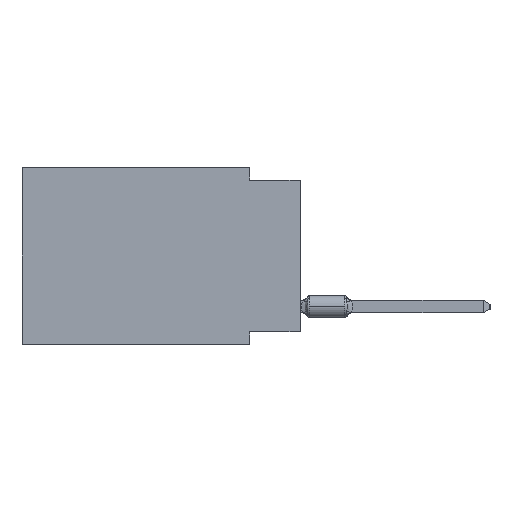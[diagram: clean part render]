
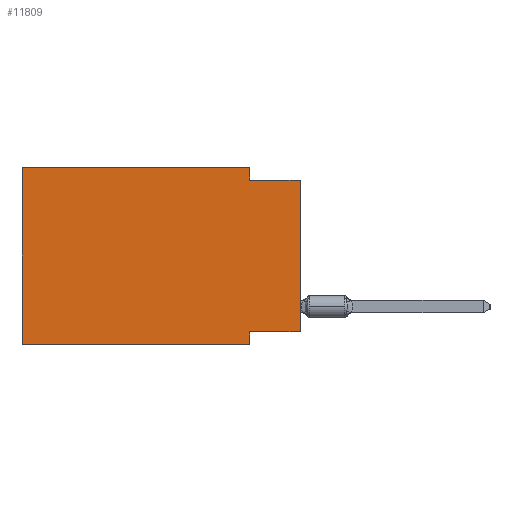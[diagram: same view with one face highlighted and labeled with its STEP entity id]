
A CAD part, left-side view. The second image highlights one B-rep face of the part: STEP entity #11809.
In plain terms, the highlighted planar face has unit normal (-1, 0, 0).
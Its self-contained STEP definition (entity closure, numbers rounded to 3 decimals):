
#423 = VECTOR ( 'NONE', #34263, 1000. ) ;
#4554 = CARTESIAN_POINT ( 'NONE',  ( 0., 2.54, -0.635 ) ) ;
#5944 = CARTESIAN_POINT ( 'NONE',  ( 0., 0., -8.255 ) ) ;
#6175 = VERTEX_POINT ( 'NONE', #35856 ) ;
#7278 = DIRECTION ( 'NONE',  ( 1., 0., 0. ) ) ;
#7930 = CARTESIAN_POINT ( 'NONE',  ( 0., 0., 0. ) ) ;
#10814 = CARTESIAN_POINT ( 'NONE',  ( 0., 13.97, 0. ) ) ;
#11542 = PLANE ( 'NONE',  #63949 ) ;
#11809 = ADVANCED_FACE ( 'NONE', ( #55339 ), #11542, .F. ) ;
#11859 = ORIENTED_EDGE ( 'NONE', *, *, #68750, .T. ) ;
#13327 = DIRECTION ( 'NONE',  ( 0., -1., 0. ) ) ;
#14011 = CARTESIAN_POINT ( 'NONE',  ( 0., 2.54, -8.89 ) ) ;
#14726 = VERTEX_POINT ( 'NONE', #75364 ) ;
#15876 = VECTOR ( 'NONE', #23024, 1000. ) ;
#18136 = VERTEX_POINT ( 'NONE', #66892 ) ;
#18162 = EDGE_CURVE ( 'NONE', #73712, #54810, #82327, .T. ) ;
#18544 = EDGE_CURVE ( 'NONE', #6175, #18136, #63864, .T. ) ;
#19356 = ORIENTED_EDGE ( 'NONE', *, *, #59135, .F. ) ;
#19653 = CARTESIAN_POINT ( 'NONE',  ( 0., 2.54, 0. ) ) ;
#20733 = VECTOR ( 'NONE', #71920, 1000. ) ;
#21104 = CARTESIAN_POINT ( 'NONE',  ( 0., 13.97, 0. ) ) ;
#21625 = VERTEX_POINT ( 'NONE', #33904 ) ;
#22103 = LINE ( 'NONE', #7930, #15876 ) ;
#22720 = CARTESIAN_POINT ( 'NONE',  ( 0., 2.54, 0. ) ) ;
#23024 = DIRECTION ( 'NONE',  ( 0., 0., 1. ) ) ;
#26619 = EDGE_CURVE ( 'NONE', #26950, #73712, #61394, .T. ) ;
#26950 = VERTEX_POINT ( 'NONE', #10814 ) ;
#27427 = CARTESIAN_POINT ( 'NONE',  ( 0., 13.97, 0. ) ) ;
#28576 = VECTOR ( 'NONE', #75507, 1000. ) ;
#33072 = VECTOR ( 'NONE', #49241, 1000. ) ;
#33843 = LINE ( 'NONE', #5944, #68025 ) ;
#33904 = CARTESIAN_POINT ( 'NONE',  ( 0., 13.97, -8.89 ) ) ;
#34263 = DIRECTION ( 'NONE',  ( 0., 0., -1. ) ) ;
#35721 = ORIENTED_EDGE ( 'NONE', *, *, #18162, .F. ) ;
#35856 = CARTESIAN_POINT ( 'NONE',  ( 0., 2.54, -8.255 ) ) ;
#38516 = VECTOR ( 'NONE', #90359, 1000. ) ;
#39804 = CARTESIAN_POINT ( 'NONE',  ( 0., 13.97, 0. ) ) ;
#40268 = LINE ( 'NONE', #39804, #28576 ) ;
#48632 = ORIENTED_EDGE ( 'NONE', *, *, #78523, .F. ) ;
#49241 = DIRECTION ( 'NONE',  ( 0., 0., -1. ) ) ;
#52419 = EDGE_CURVE ( 'NONE', #14726, #77624, #22103, .T. ) ;
#54810 = VERTEX_POINT ( 'NONE', #4554 ) ;
#55339 = FACE_OUTER_BOUND ( 'NONE', #86057, .T. ) ;
#57518 = VECTOR ( 'NONE', #13327, 1000. ) ;
#59098 = EDGE_CURVE ( 'NONE', #14726, #6175, #33843, .T. ) ;
#59135 = EDGE_CURVE ( 'NONE', #21625, #26950, #40268, .T. ) ;
#59907 = CARTESIAN_POINT ( 'NONE',  ( 0., 0., -0.635 ) ) ;
#60044 = DIRECTION ( 'NONE',  ( 0., 0., -1. ) ) ;
#61062 = CARTESIAN_POINT ( 'NONE',  ( 0., 13.97, -8.89 ) ) ;
#61394 = LINE ( 'NONE', #21104, #57518 ) ;
#63864 = LINE ( 'NONE', #14011, #33072 ) ;
#63949 = AXIS2_PLACEMENT_3D ( 'NONE', #27427, #7278, #60044 ) ;
#66892 = CARTESIAN_POINT ( 'NONE',  ( 0., 2.54, -8.89 ) ) ;
#67141 = ORIENTED_EDGE ( 'NONE', *, *, #18544, .F. ) ;
#68025 = VECTOR ( 'NONE', #87881, 1000. ) ;
#68750 = EDGE_CURVE ( 'NONE', #21625, #18136, #81189, .T. ) ;
#71600 = CARTESIAN_POINT ( 'NONE',  ( 0., 0., -0.635 ) ) ;
#71920 = DIRECTION ( 'NONE',  ( 0., -1., 0. ) ) ;
#73712 = VERTEX_POINT ( 'NONE', #22720 ) ;
#75364 = CARTESIAN_POINT ( 'NONE',  ( 0., 0., -8.255 ) ) ;
#75507 = DIRECTION ( 'NONE',  ( 0., 0., 1. ) ) ;
#77624 = VERTEX_POINT ( 'NONE', #71600 ) ;
#78523 = EDGE_CURVE ( 'NONE', #54810, #77624, #85688, .T. ) ;
#81189 = LINE ( 'NONE', #61062, #38516 ) ;
#82327 = LINE ( 'NONE', #19653, #423 ) ;
#85688 = LINE ( 'NONE', #59907, #20733 ) ;
#86057 = EDGE_LOOP ( 'NONE', ( #87272, #48632, #35721, #86935, #19356, #11859, #67141, #90285 ) ) ;
#86935 = ORIENTED_EDGE ( 'NONE', *, *, #26619, .F. ) ;
#87272 = ORIENTED_EDGE ( 'NONE', *, *, #52419, .T. ) ;
#87881 = DIRECTION ( 'NONE',  ( 0., 1., 0. ) ) ;
#90285 = ORIENTED_EDGE ( 'NONE', *, *, #59098, .F. ) ;
#90359 = DIRECTION ( 'NONE',  ( 0., -1., 0. ) ) ;
